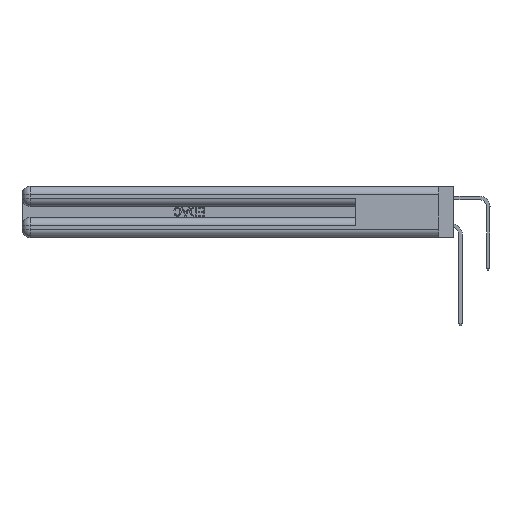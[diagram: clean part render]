
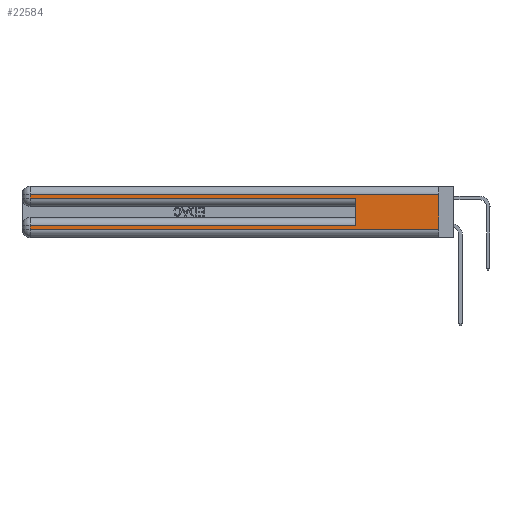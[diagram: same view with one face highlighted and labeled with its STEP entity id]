
A CAD part, left-side view. The second image highlights one B-rep face of the part: STEP entity #22584.
In plain terms, the highlighted planar face has unit normal (-1, 0, 0).
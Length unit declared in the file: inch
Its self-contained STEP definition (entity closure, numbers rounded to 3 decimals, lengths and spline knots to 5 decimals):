
#522 = VECTOR ( 'NONE', #36965, 39.37008 ) ;
#1324 = VECTOR ( 'NONE', #21000, 39.37008 ) ;
#1548 = CARTESIAN_POINT ( 'NONE',  ( 0., 2.94, 0.085 ) ) ;
#2660 = CARTESIAN_POINT ( 'NONE',  ( 0., 0., 0.31 ) ) ;
#2841 = ORIENTED_EDGE ( 'NONE', *, *, #5111, .F. ) ;
#2931 = VECTOR ( 'NONE', #38055, 39.37008 ) ;
#3348 = CARTESIAN_POINT ( 'NONE',  ( 0., 2.94, 0.31 ) ) ;
#4258 = LINE ( 'NONE', #13062, #21975 ) ;
#4658 = CARTESIAN_POINT ( 'NONE',  ( 0., 0., 0.37 ) ) ;
#5055 = DIRECTION ( 'NONE',  ( 0., 0., -1. ) ) ;
#5111 = EDGE_CURVE ( 'NONE', #33819, #35262, #35432, .T. ) ;
#5227 = VECTOR ( 'NONE', #20855, 39.37008 ) ;
#5600 = ORIENTED_EDGE ( 'NONE', *, *, #38378, .T. ) ;
#6870 = CARTESIAN_POINT ( 'NONE',  ( 0., 2.94, 0.285 ) ) ;
#6898 = LINE ( 'NONE', #33154, #522 ) ;
#10230 = EDGE_CURVE ( 'NONE', #33082, #11920, #36454, .T. ) ;
#10937 = AXIS2_PLACEMENT_3D ( 'NONE', #4658, #41179, #45985 ) ;
#10943 = ORIENTED_EDGE ( 'NONE', *, *, #10230, .T. ) ;
#11595 = VECTOR ( 'NONE', #20593, 39.37008 ) ;
#11920 = VERTEX_POINT ( 'NONE', #1548 ) ;
#12560 = DIRECTION ( 'NONE',  ( 0., 0., -1. ) ) ;
#13062 = CARTESIAN_POINT ( 'NONE',  ( 0., 2.94, 0.37 ) ) ;
#13321 = CARTESIAN_POINT ( 'NONE',  ( 0., 0.6, 0.285 ) ) ;
#14383 = EDGE_CURVE ( 'NONE', #28722, #18335, #25590, .T. ) ;
#14635 = CARTESIAN_POINT ( 'NONE',  ( 0., 0., 0.31 ) ) ;
#17225 = LINE ( 'NONE', #21309, #5227 ) ;
#18335 = VERTEX_POINT ( 'NONE', #6870 ) ;
#19298 = CARTESIAN_POINT ( 'NONE',  ( 0., 0., 0.06 ) ) ;
#19876 = VECTOR ( 'NONE', #28119, 39.37008 ) ;
#20283 = FACE_OUTER_BOUND ( 'NONE', #38263, .T. ) ;
#20593 = DIRECTION ( 'NONE',  ( 0., -1., 0. ) ) ;
#20855 = DIRECTION ( 'NONE',  ( 0., 0., 1. ) ) ;
#21000 = DIRECTION ( 'NONE',  ( 0., 0., -1. ) ) ;
#21309 = CARTESIAN_POINT ( 'NONE',  ( 0., 0.6, 0.145 ) ) ;
#21782 = ORIENTED_EDGE ( 'NONE', *, *, #14383, .T. ) ;
#21975 = VECTOR ( 'NONE', #12560, 39.37008 ) ;
#22377 = LINE ( 'NONE', #31373, #11595 ) ;
#22584 = ADVANCED_FACE ( 'NONE', ( #20283 ), #37528, .F. ) ;
#22668 = LINE ( 'NONE', #2660, #19876 ) ;
#25176 = EDGE_CURVE ( 'NONE', #18335, #31721, #6898, .T. ) ;
#25440 = EDGE_CURVE ( 'NONE', #11920, #43595, #4258, .T. ) ;
#25590 = LINE ( 'NONE', #45091, #39214 ) ;
#28119 = DIRECTION ( 'NONE',  ( 0., 1., 0. ) ) ;
#28722 = VERTEX_POINT ( 'NONE', #3348 ) ;
#29838 = CARTESIAN_POINT ( 'NONE',  ( 0., 2.94, 0.06 ) ) ;
#30381 = ORIENTED_EDGE ( 'NONE', *, *, #25176, .T. ) ;
#31092 = EDGE_CURVE ( 'NONE', #33819, #28722, #22668, .T. ) ;
#31373 = CARTESIAN_POINT ( 'NONE',  ( 0., 0., 0.06 ) ) ;
#31721 = VERTEX_POINT ( 'NONE', #13321 ) ;
#33082 = VERTEX_POINT ( 'NONE', #39288 ) ;
#33154 = CARTESIAN_POINT ( 'NONE',  ( 0., 0., 0.285 ) ) ;
#33819 = VERTEX_POINT ( 'NONE', #14635 ) ;
#35262 = VERTEX_POINT ( 'NONE', #19298 ) ;
#35432 = LINE ( 'NONE', #37782, #1324 ) ;
#36454 = LINE ( 'NONE', #39845, #2931 ) ;
#36663 = ORIENTED_EDGE ( 'NONE', *, *, #41792, .F. ) ;
#36684 = ORIENTED_EDGE ( 'NONE', *, *, #31092, .T. ) ;
#36965 = DIRECTION ( 'NONE',  ( 0., -1., 0. ) ) ;
#37528 = PLANE ( 'NONE',  #10937 ) ;
#37782 = CARTESIAN_POINT ( 'NONE',  ( 0., 0., 0.37 ) ) ;
#38055 = DIRECTION ( 'NONE',  ( 0., 1., 0. ) ) ;
#38263 = EDGE_LOOP ( 'NONE', ( #2841, #36684, #21782, #30381, #36663, #10943, #43730, #5600 ) ) ;
#38378 = EDGE_CURVE ( 'NONE', #43595, #35262, #22377, .T. ) ;
#39214 = VECTOR ( 'NONE', #5055, 39.37008 ) ;
#39288 = CARTESIAN_POINT ( 'NONE',  ( 0., 0.6, 0.085 ) ) ;
#39845 = CARTESIAN_POINT ( 'NONE',  ( 0., 0., 0.085 ) ) ;
#41179 = DIRECTION ( 'NONE',  ( 1., 0., 0. ) ) ;
#41792 = EDGE_CURVE ( 'NONE', #33082, #31721, #17225, .T. ) ;
#43595 = VERTEX_POINT ( 'NONE', #29838 ) ;
#43730 = ORIENTED_EDGE ( 'NONE', *, *, #25440, .T. ) ;
#45091 = CARTESIAN_POINT ( 'NONE',  ( 0., 2.94, 0.37 ) ) ;
#45985 = DIRECTION ( 'NONE',  ( 0., 0., -1. ) ) ;
